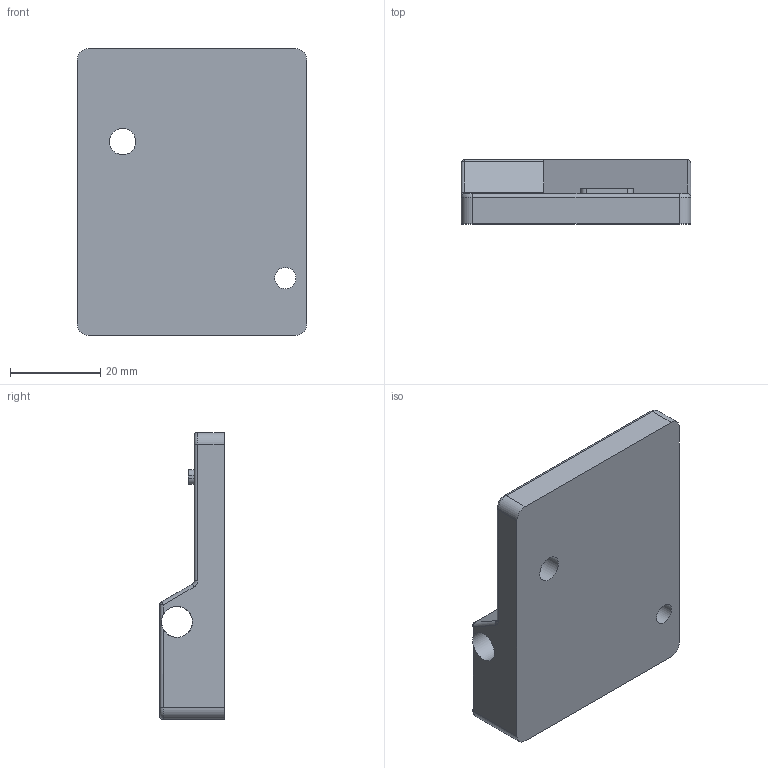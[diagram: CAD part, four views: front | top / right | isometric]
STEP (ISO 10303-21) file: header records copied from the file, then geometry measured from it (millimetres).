
FILE_DESCRIPTION( ( '' ), ' ' );
FILE_NAME( '5a114dfda6a9fe0be5a87cf2.step', '2017-11-19T09:25:17', ( '' ), ( '' ), ' ', ' ', ' ' );
FILE_SCHEMA( ( 'AUTOMOTIVE_DESIGN { 1 0 10303 214 1 1 1 1 }' ) );
Length unit declared in the file: metre
Products named in the file (1): Part 1
Bounding box: 50.8 x 14.29 x 63.5 mm (x, y, z)
Volume: 27545 mm3; surface area: 10058 mm2
Topology: 1 solids, 1 shells, 62 faces, 164 edges, 105 vertices
Faces by surface type: plane 34, cylinder 22, torus 5, sphere 1
Full cylindrical faces by diameter (mm): 4.699 x1, 5.842 x1, 6.35 x1, 6.858 x1
Entity records: 2399 total; most frequent: CARTESIAN_POINT 333, DIRECTION 331, ORIENTED_EDGE 314, EDGE_CURVE 157, AXIS2_PLACEMENT_3D 112, LINE 107, VECTOR 107, VERTEX_POINT 102
